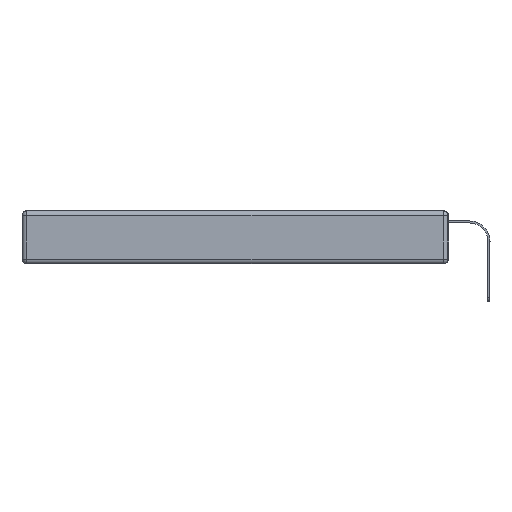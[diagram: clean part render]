
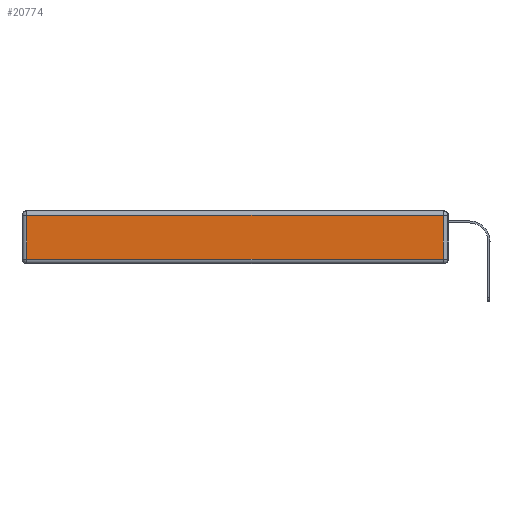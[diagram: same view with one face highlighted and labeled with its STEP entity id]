
A CAD part, left-side view. The second image highlights one B-rep face of the part: STEP entity #20774.
In plain terms, the highlighted planar face has unit normal (-1, 0, 0).
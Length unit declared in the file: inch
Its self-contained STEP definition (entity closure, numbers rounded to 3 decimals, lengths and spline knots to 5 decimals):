
#886 = CARTESIAN_POINT ( 'NONE',  ( 0., 2.72, -0.313 ) ) ;
#2467 = VECTOR ( 'NONE', #14616, 39.37008 ) ;
#3022 = ORIENTED_EDGE ( 'NONE', *, *, #6446, .T. ) ;
#3121 = CARTESIAN_POINT ( 'NONE',  ( 0., 0., -0.313 ) ) ;
#3473 = LINE ( 'NONE', #20958, #7012 ) ;
#4809 = VECTOR ( 'NONE', #11591, 39.37008 ) ;
#5602 = DIRECTION ( 'NONE',  ( 0., 0., 1. ) ) ;
#6023 = DIRECTION ( 'NONE',  ( 0., 0., 1. ) ) ;
#6446 = EDGE_CURVE ( 'NONE', #16959, #16140, #21499, .T. ) ;
#7012 = VECTOR ( 'NONE', #5602, 39.37008 ) ;
#7448 = LINE ( 'NONE', #18168, #24925 ) ;
#8268 = DIRECTION ( 'NONE',  ( -1., 0., 0. ) ) ;
#8788 = ORIENTED_EDGE ( 'NONE', *, *, #22850, .T. ) ;
#9683 = ORIENTED_EDGE ( 'NONE', *, *, #21945, .T. ) ;
#10962 = CARTESIAN_POINT ( 'NONE',  ( 0., 0.03, -0.03 ) ) ;
#11591 = DIRECTION ( 'NONE',  ( 0., -1., 0. ) ) ;
#12090 = DIRECTION ( 'NONE',  ( 0., 1., 0. ) ) ;
#13129 = VERTEX_POINT ( 'NONE', #10962 ) ;
#14485 = CARTESIAN_POINT ( 'NONE',  ( 0., 0.03, -0.313 ) ) ;
#14616 = DIRECTION ( 'NONE',  ( 0., 0., -1. ) ) ;
#15037 = PLANE ( 'NONE',  #21367 ) ;
#15691 = EDGE_LOOP ( 'NONE', ( #8788, #9683, #22271, #3022 ) ) ;
#16140 = VERTEX_POINT ( 'NONE', #886 ) ;
#16692 = EDGE_CURVE ( 'NONE', #13129, #16959, #7448, .T. ) ;
#16959 = VERTEX_POINT ( 'NONE', #19688 ) ;
#18168 = CARTESIAN_POINT ( 'NONE',  ( 0., 2.75, -0.03 ) ) ;
#19688 = CARTESIAN_POINT ( 'NONE',  ( 0., 2.72, -0.03 ) ) ;
#20774 = ADVANCED_FACE ( 'NONE', ( #23331 ), #15037, .T. ) ;
#20958 = CARTESIAN_POINT ( 'NONE',  ( 0., 0.03, -0.343 ) ) ;
#21363 = CARTESIAN_POINT ( 'NONE',  ( 0., 0., -0.343 ) ) ;
#21367 = AXIS2_PLACEMENT_3D ( 'NONE', #21363, #8268, #6023 ) ;
#21499 = LINE ( 'NONE', #23602, #2467 ) ;
#21945 = EDGE_CURVE ( 'NONE', #24663, #13129, #3473, .T. ) ;
#22271 = ORIENTED_EDGE ( 'NONE', *, *, #16692, .T. ) ;
#22707 = LINE ( 'NONE', #3121, #4809 ) ;
#22850 = EDGE_CURVE ( 'NONE', #16140, #24663, #22707, .T. ) ;
#23331 = FACE_OUTER_BOUND ( 'NONE', #15691, .T. ) ;
#23602 = CARTESIAN_POINT ( 'NONE',  ( 0., 2.72, -0.343 ) ) ;
#24663 = VERTEX_POINT ( 'NONE', #14485 ) ;
#24925 = VECTOR ( 'NONE', #12090, 39.37008 ) ;
